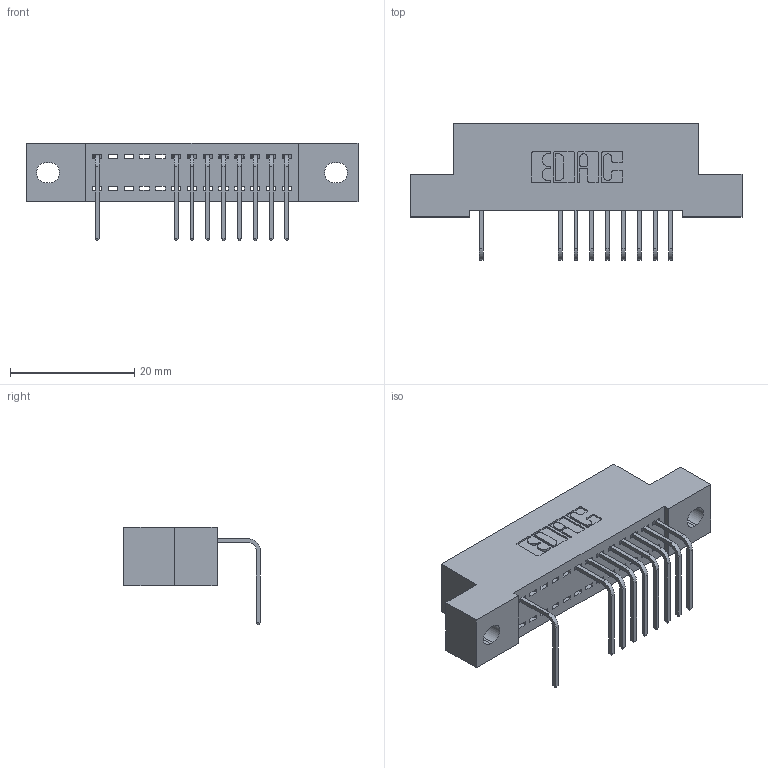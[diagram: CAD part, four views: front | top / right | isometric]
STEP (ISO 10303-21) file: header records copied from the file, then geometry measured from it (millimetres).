
FILE_DESCRIPTION (( 'STEP AP203' ), '1' );
FILE_NAME ('342-013-558-102.STEP', '2018-08-10T16:33:19', ( '' ), ( '' ), 'SwSTEP 2.0', 'SolidWorks 2016', '' );
FILE_SCHEMA (( 'CONFIG_CONTROL_DESIGN' ));
Length unit declared in the file: inch
Products named in the file (3): 345-292-001_558 Tail - 2; 342-013-558-102; 342 Part_.128 Slot
Assembly tree (10 placements, depth 2):
  342-013-558-102
    342 Part_.128 Slot
    345-292-001_558 Tail - 2  x9
Bounding box: 53.34 x 21.91 x 15.62 mm (x, y, z)
Volume: 4502.1 mm3; surface area: 5762.6 mm2
Topology: 10 solids, 10 shells, 702 faces, 2117 edges, 1398 vertices
Faces by surface type: plane 514, cylinder 188
Entity records: 11657 total; most frequent: CARTESIAN_POINT 2041, ORIENTED_EDGE 1994, DIRECTION 1775, EDGE_CURVE 997, VECTOR 869, LINE 869, VERTEX_POINT 662, AXIS2_PLACEMENT_3D 453
